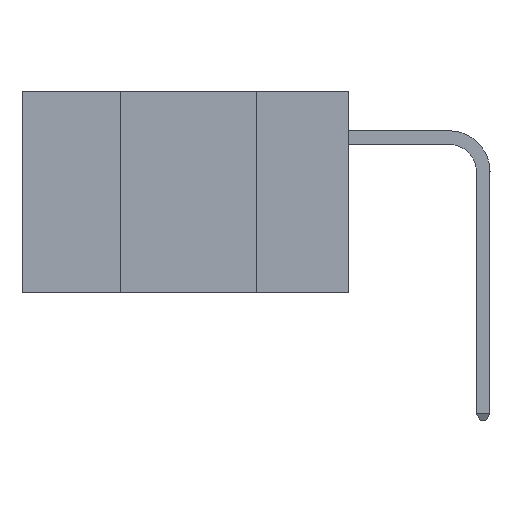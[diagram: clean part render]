
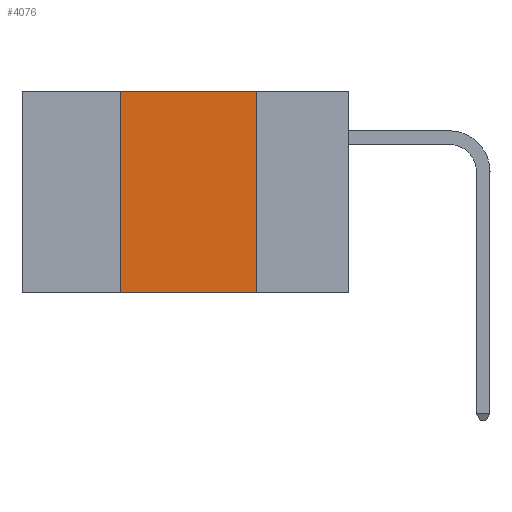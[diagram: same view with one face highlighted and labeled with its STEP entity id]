
A CAD part, left-side view. The second image highlights one B-rep face of the part: STEP entity #4076.
In plain terms, the highlighted planar face has unit normal (-1, 0, 0).
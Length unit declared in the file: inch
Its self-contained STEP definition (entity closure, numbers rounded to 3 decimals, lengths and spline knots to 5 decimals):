
#63 = CARTESIAN_POINT ( 'NONE',  ( 0., 0.17, 0. ) ) ;
#648 = ORIENTED_EDGE ( 'NONE', *, *, #4964, .F. ) ;
#1129 = CARTESIAN_POINT ( 'NONE',  ( 0., 0.42, 0. ) ) ;
#1260 = VERTEX_POINT ( 'NONE', #2532 ) ;
#1328 = ORIENTED_EDGE ( 'NONE', *, *, #1492, .T. ) ;
#1492 = EDGE_CURVE ( 'NONE', #4348, #3577, #8232, .T. ) ;
#1685 = DIRECTION ( 'NONE',  ( 0., 0., -1. ) ) ;
#1796 = CARTESIAN_POINT ( 'NONE',  ( 0., 0.42, 0. ) ) ;
#1799 = VERTEX_POINT ( 'NONE', #1796 ) ;
#1868 = FACE_OUTER_BOUND ( 'NONE', #8171, .T. ) ;
#1902 = CARTESIAN_POINT ( 'NONE',  ( 0., 0.17, -0.37 ) ) ;
#2123 = DIRECTION ( 'NONE',  ( 0., 0., -1. ) ) ;
#2282 = LINE ( 'NONE', #1129, #7108 ) ;
#2532 = CARTESIAN_POINT ( 'NONE',  ( 0., 0.17, 0. ) ) ;
#2657 = CARTESIAN_POINT ( 'NONE',  ( 0., 0.6, -0.37 ) ) ;
#2739 = DIRECTION ( 'NONE',  ( 0., 0., 1. ) ) ;
#2745 = VECTOR ( 'NONE', #3369, 39.37008 ) ;
#3369 = DIRECTION ( 'NONE',  ( 0., -1., 0. ) ) ;
#3430 = AXIS2_PLACEMENT_3D ( 'NONE', #5171, #6880, #2123 ) ;
#3577 = VERTEX_POINT ( 'NONE', #1902 ) ;
#3622 = EDGE_CURVE ( 'NONE', #4348, #1799, #2282, .T. ) ;
#3966 = VECTOR ( 'NONE', #8347, 39.37008 ) ;
#4076 = ADVANCED_FACE ( 'NONE', ( #1868 ), #8098, .F. ) ;
#4117 = ORIENTED_EDGE ( 'NONE', *, *, #3622, .F. ) ;
#4216 = CARTESIAN_POINT ( 'NONE',  ( 0., 0.6, 0. ) ) ;
#4348 = VERTEX_POINT ( 'NONE', #8895 ) ;
#4964 = EDGE_CURVE ( 'NONE', #1260, #3577, #7512, .T. ) ;
#5171 = CARTESIAN_POINT ( 'NONE',  ( 0., 0.6, 0. ) ) ;
#5511 = VECTOR ( 'NONE', #1685, 39.37008 ) ;
#6221 = LINE ( 'NONE', #4216, #3966 ) ;
#6480 = ORIENTED_EDGE ( 'NONE', *, *, #8592, .F. ) ;
#6880 = DIRECTION ( 'NONE',  ( 1., 0., 0. ) ) ;
#7108 = VECTOR ( 'NONE', #2739, 39.37008 ) ;
#7512 = LINE ( 'NONE', #63, #5511 ) ;
#8098 = PLANE ( 'NONE',  #3430 ) ;
#8171 = EDGE_LOOP ( 'NONE', ( #648, #6480, #4117, #1328 ) ) ;
#8232 = LINE ( 'NONE', #2657, #2745 ) ;
#8347 = DIRECTION ( 'NONE',  ( 0., -1., 0. ) ) ;
#8592 = EDGE_CURVE ( 'NONE', #1799, #1260, #6221, .T. ) ;
#8895 = CARTESIAN_POINT ( 'NONE',  ( 0., 0.42, -0.37 ) ) ;
